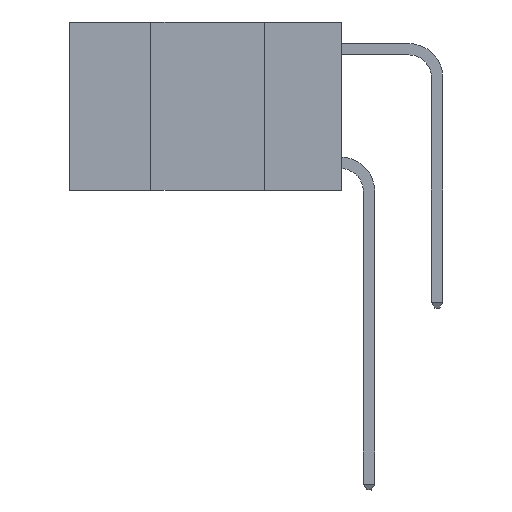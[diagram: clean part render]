
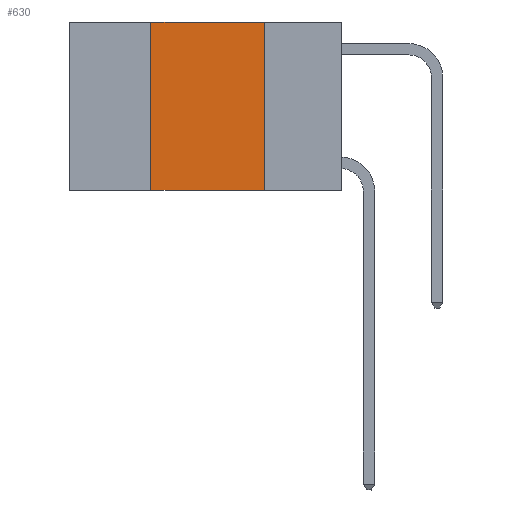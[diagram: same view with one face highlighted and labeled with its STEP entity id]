
A CAD part, left-side view. The second image highlights one B-rep face of the part: STEP entity #630.
In plain terms, the highlighted planar face has unit normal (-1, 0, 0).
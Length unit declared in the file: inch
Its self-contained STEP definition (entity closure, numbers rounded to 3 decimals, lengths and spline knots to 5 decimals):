
#310 = DIRECTION ( 'NONE',  ( 0., 0., -1. ) ) ;
#630 = ADVANCED_FACE ( 'NONE', ( #13574 ), #8768, .F. ) ;
#693 = VECTOR ( 'NONE', #5500, 39.37008 ) ;
#726 = DIRECTION ( 'NONE',  ( 0., 0., -1. ) ) ;
#1225 = ORIENTED_EDGE ( 'NONE', *, *, #4437, .F. ) ;
#1424 = CARTESIAN_POINT ( 'NONE',  ( 0., 0.6, 0. ) ) ;
#2168 = VERTEX_POINT ( 'NONE', #3463 ) ;
#3463 = CARTESIAN_POINT ( 'NONE',  ( 0., 0.42, 0. ) ) ;
#3475 = AXIS2_PLACEMENT_3D ( 'NONE', #10763, #12776, #726 ) ;
#4220 = VECTOR ( 'NONE', #20376, 39.37008 ) ;
#4437 = EDGE_CURVE ( 'NONE', #11164, #2168, #9625, .T. ) ;
#4842 = EDGE_CURVE ( 'NONE', #11164, #4879, #11434, .T. ) ;
#4879 = VERTEX_POINT ( 'NONE', #9585 ) ;
#5331 = ORIENTED_EDGE ( 'NONE', *, *, #15198, .F. ) ;
#5500 = DIRECTION ( 'NONE',  ( 0., -1., 0. ) ) ;
#6615 = ORIENTED_EDGE ( 'NONE', *, *, #4842, .T. ) ;
#7481 = CARTESIAN_POINT ( 'NONE',  ( 0., 0.6, -0.37 ) ) ;
#7823 = LINE ( 'NONE', #8445, #17788 ) ;
#8445 = CARTESIAN_POINT ( 'NONE',  ( 0., 0.17, 0. ) ) ;
#8768 = PLANE ( 'NONE',  #3475 ) ;
#9585 = CARTESIAN_POINT ( 'NONE',  ( 0., 0.17, -0.37 ) ) ;
#9625 = LINE ( 'NONE', #18292, #4220 ) ;
#10688 = ORIENTED_EDGE ( 'NONE', *, *, #20642, .F. ) ;
#10763 = CARTESIAN_POINT ( 'NONE',  ( 0., 0.6, 0. ) ) ;
#11164 = VERTEX_POINT ( 'NONE', #18266 ) ;
#11434 = LINE ( 'NONE', #7481, #16754 ) ;
#12776 = DIRECTION ( 'NONE',  ( 1., 0., 0. ) ) ;
#13360 = CARTESIAN_POINT ( 'NONE',  ( 0., 0.17, 0. ) ) ;
#13574 = FACE_OUTER_BOUND ( 'NONE', #24973, .T. ) ;
#15198 = EDGE_CURVE ( 'NONE', #19915, #4879, #7823, .T. ) ;
#16754 = VECTOR ( 'NONE', #25381, 39.37008 ) ;
#17788 = VECTOR ( 'NONE', #310, 39.37008 ) ;
#18266 = CARTESIAN_POINT ( 'NONE',  ( 0., 0.42, -0.37 ) ) ;
#18292 = CARTESIAN_POINT ( 'NONE',  ( 0., 0.42, 0. ) ) ;
#19915 = VERTEX_POINT ( 'NONE', #13360 ) ;
#20376 = DIRECTION ( 'NONE',  ( 0., 0., 1. ) ) ;
#20642 = EDGE_CURVE ( 'NONE', #2168, #19915, #22579, .T. ) ;
#22579 = LINE ( 'NONE', #1424, #693 ) ;
#24973 = EDGE_LOOP ( 'NONE', ( #5331, #10688, #1225, #6615 ) ) ;
#25381 = DIRECTION ( 'NONE',  ( 0., -1., 0. ) ) ;
